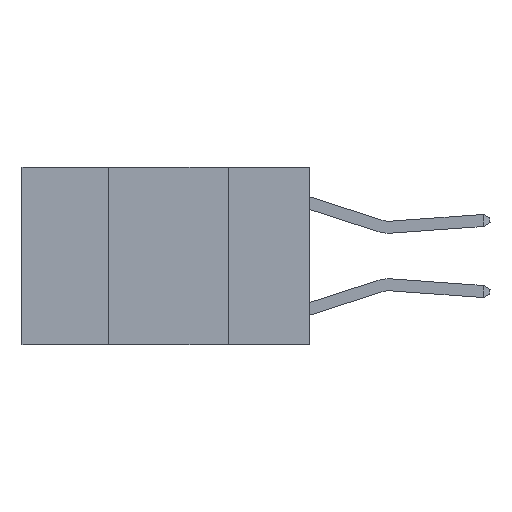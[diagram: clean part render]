
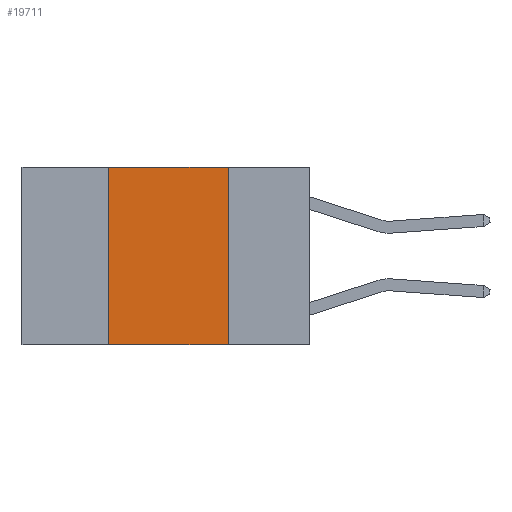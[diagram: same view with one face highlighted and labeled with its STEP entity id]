
A CAD part, left-side view. The second image highlights one B-rep face of the part: STEP entity #19711.
In plain terms, the highlighted planar face has unit normal (-1, 0, 0).
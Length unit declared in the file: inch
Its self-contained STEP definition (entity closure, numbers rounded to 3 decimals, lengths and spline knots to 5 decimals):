
#791 = LINE ( 'NONE', #8849, #16924 ) ;
#1934 = CARTESIAN_POINT ( 'NONE',  ( 0., 0.6, -0.37 ) ) ;
#4250 = VERTEX_POINT ( 'NONE', #14651 ) ;
#4615 = LINE ( 'NONE', #23289, #5028 ) ;
#4705 = ORIENTED_EDGE ( 'NONE', *, *, #7878, .T. ) ;
#5028 = VECTOR ( 'NONE', #23652, 39.37008 ) ;
#5676 = DIRECTION ( 'NONE',  ( 1., 0., 0. ) ) ;
#5777 = DIRECTION ( 'NONE',  ( 0., -1., 0. ) ) ;
#7759 = LINE ( 'NONE', #1934, #16013 ) ;
#7878 = EDGE_CURVE ( 'NONE', #8851, #12561, #7759, .T. ) ;
#8849 = CARTESIAN_POINT ( 'NONE',  ( 0., 0.42, 0. ) ) ;
#8851 = VERTEX_POINT ( 'NONE', #11217 ) ;
#9518 = CARTESIAN_POINT ( 'NONE',  ( 0., 0.6, 0. ) ) ;
#9619 = CARTESIAN_POINT ( 'NONE',  ( 0., 0.6, 0. ) ) ;
#9633 = DIRECTION ( 'NONE',  ( 0., -1., 0. ) ) ;
#10071 = VERTEX_POINT ( 'NONE', #14827 ) ;
#10247 = ORIENTED_EDGE ( 'NONE', *, *, #16703, .F. ) ;
#11217 = CARTESIAN_POINT ( 'NONE',  ( 0., 0.42, -0.37 ) ) ;
#11475 = LINE ( 'NONE', #9518, #13512 ) ;
#12561 = VERTEX_POINT ( 'NONE', #22826 ) ;
#13512 = VECTOR ( 'NONE', #9633, 39.37008 ) ;
#14651 = CARTESIAN_POINT ( 'NONE',  ( 0., 0.17, 0. ) ) ;
#14711 = ORIENTED_EDGE ( 'NONE', *, *, #23597, .F. ) ;
#14827 = CARTESIAN_POINT ( 'NONE',  ( 0., 0.42, 0. ) ) ;
#15060 = PLANE ( 'NONE',  #17999 ) ;
#16013 = VECTOR ( 'NONE', #5777, 39.37008 ) ;
#16028 = ORIENTED_EDGE ( 'NONE', *, *, #24376, .F. ) ;
#16622 = EDGE_LOOP ( 'NONE', ( #14711, #10247, #16028, #4705 ) ) ;
#16703 = EDGE_CURVE ( 'NONE', #10071, #4250, #11475, .T. ) ;
#16924 = VECTOR ( 'NONE', #18117, 39.37008 ) ;
#17999 = AXIS2_PLACEMENT_3D ( 'NONE', #9619, #5676, #18779 ) ;
#18117 = DIRECTION ( 'NONE',  ( 0., 0., 1. ) ) ;
#18779 = DIRECTION ( 'NONE',  ( 0., 0., -1. ) ) ;
#19711 = ADVANCED_FACE ( 'NONE', ( #20657 ), #15060, .F. ) ;
#20657 = FACE_OUTER_BOUND ( 'NONE', #16622, .T. ) ;
#22826 = CARTESIAN_POINT ( 'NONE',  ( 0., 0.17, -0.37 ) ) ;
#23289 = CARTESIAN_POINT ( 'NONE',  ( 0., 0.17, 0. ) ) ;
#23597 = EDGE_CURVE ( 'NONE', #4250, #12561, #4615, .T. ) ;
#23652 = DIRECTION ( 'NONE',  ( 0., 0., -1. ) ) ;
#24376 = EDGE_CURVE ( 'NONE', #8851, #10071, #791, .T. ) ;
